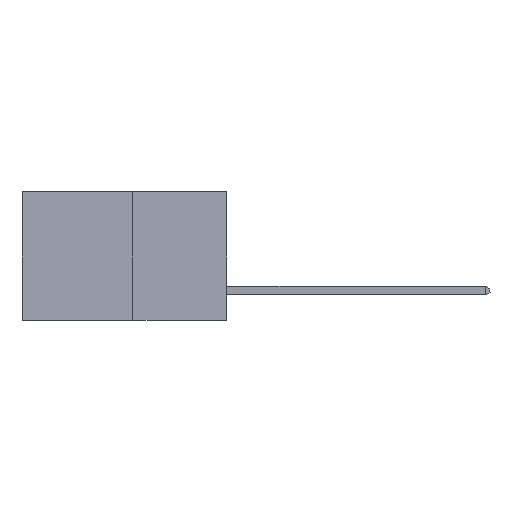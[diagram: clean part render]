
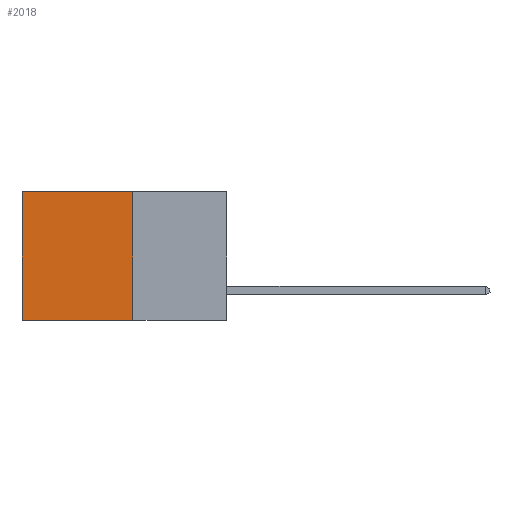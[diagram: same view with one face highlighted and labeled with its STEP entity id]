
A CAD part, left-side view. The second image highlights one B-rep face of the part: STEP entity #2018.
In plain terms, the highlighted planar face has unit normal (-1, 0, 0).
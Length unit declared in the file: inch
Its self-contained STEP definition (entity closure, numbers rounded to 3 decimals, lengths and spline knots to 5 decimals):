
#318 = VERTEX_POINT ( 'NONE', #12639 ) ;
#390 = DIRECTION ( 'NONE',  ( 0., 1., 0. ) ) ;
#492 = LINE ( 'NONE', #8489, #8615 ) ;
#612 = VERTEX_POINT ( 'NONE', #4420 ) ;
#912 = DIRECTION ( 'NONE',  ( 0., 0., -1. ) ) ;
#2018 = ADVANCED_FACE ( 'NONE', ( #14347 ), #11362, .F. ) ;
#2123 = VECTOR ( 'NONE', #4103, 39.37008 ) ;
#2221 = VERTEX_POINT ( 'NONE', #10891 ) ;
#3073 = AXIS2_PLACEMENT_3D ( 'NONE', #10742, #11597, #9361 ) ;
#3304 = VECTOR ( 'NONE', #4096, 39.37008 ) ;
#3731 = EDGE_CURVE ( 'NONE', #5586, #2221, #6718, .T. ) ;
#4096 = DIRECTION ( 'NONE',  ( 0., 1., 0. ) ) ;
#4103 = DIRECTION ( 'NONE',  ( 0., 0., -1. ) ) ;
#4344 = ORIENTED_EDGE ( 'NONE', *, *, #12937, .T. ) ;
#4420 = CARTESIAN_POINT ( 'NONE',  ( 0.277, 0.27, -0.37 ) ) ;
#4648 = LINE ( 'NONE', #14249, #10193 ) ;
#4955 = ORIENTED_EDGE ( 'NONE', *, *, #10982, .F. ) ;
#5112 = CARTESIAN_POINT ( 'NONE',  ( 0.277, 0.27, 0. ) ) ;
#5586 = VERTEX_POINT ( 'NONE', #5112 ) ;
#5603 = LINE ( 'NONE', #9759, #2123 ) ;
#5963 = ORIENTED_EDGE ( 'NONE', *, *, #9693, .F. ) ;
#6718 = LINE ( 'NONE', #11829, #3304 ) ;
#8489 = CARTESIAN_POINT ( 'NONE',  ( 0.277, 0.27, -0.37 ) ) ;
#8615 = VECTOR ( 'NONE', #390, 39.37008 ) ;
#9361 = DIRECTION ( 'NONE',  ( 0., 0., -1. ) ) ;
#9693 = EDGE_CURVE ( 'NONE', #612, #318, #492, .T. ) ;
#9759 = CARTESIAN_POINT ( 'NONE',  ( 0.277, 0.27, -0.37 ) ) ;
#10193 = VECTOR ( 'NONE', #912, 39.37008 ) ;
#10742 = CARTESIAN_POINT ( 'NONE',  ( 0.277, 0.27, -0.37 ) ) ;
#10891 = CARTESIAN_POINT ( 'NONE',  ( 0.277, 0.59, 0. ) ) ;
#10982 = EDGE_CURVE ( 'NONE', #5586, #612, #5603, .T. ) ;
#11362 = PLANE ( 'NONE',  #3073 ) ;
#11597 = DIRECTION ( 'NONE',  ( 1., 0., 0. ) ) ;
#11638 = EDGE_LOOP ( 'NONE', ( #4344, #5963, #4955, #13443 ) ) ;
#11829 = CARTESIAN_POINT ( 'NONE',  ( 0.277, 0.27, 0. ) ) ;
#12639 = CARTESIAN_POINT ( 'NONE',  ( 0.277, 0.59, -0.37 ) ) ;
#12937 = EDGE_CURVE ( 'NONE', #2221, #318, #4648, .T. ) ;
#13443 = ORIENTED_EDGE ( 'NONE', *, *, #3731, .T. ) ;
#14249 = CARTESIAN_POINT ( 'NONE',  ( 0.277, 0.59, -0.37 ) ) ;
#14347 = FACE_OUTER_BOUND ( 'NONE', #11638, .T. ) ;
